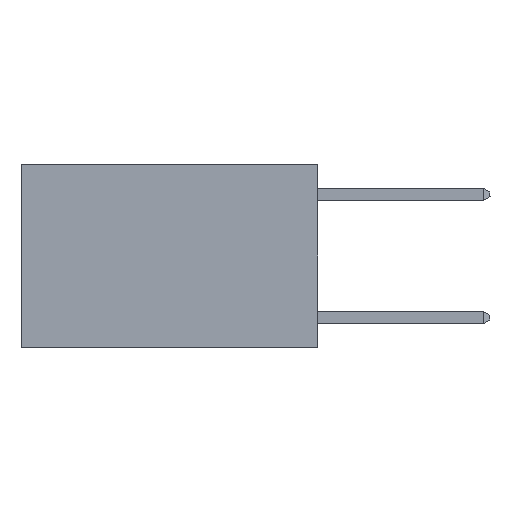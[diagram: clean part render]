
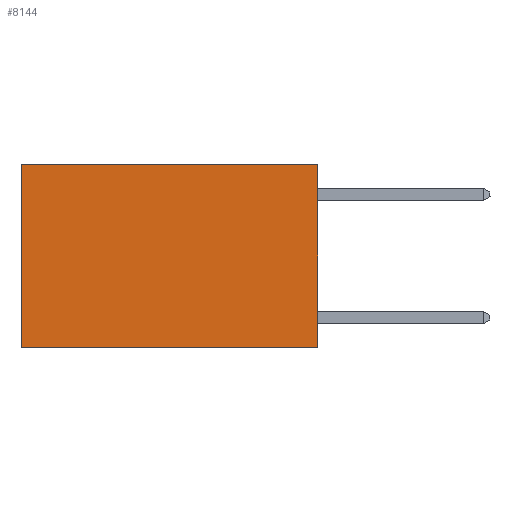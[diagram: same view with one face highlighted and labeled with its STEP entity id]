
A CAD part, left-side view. The second image highlights one B-rep face of the part: STEP entity #8144.
In plain terms, the highlighted planar face has unit normal (-1, 0, 0).
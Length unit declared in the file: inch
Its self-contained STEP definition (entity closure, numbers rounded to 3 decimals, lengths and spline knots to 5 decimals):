
#30 = CARTESIAN_POINT ( 'NONE',  ( 0.2625, 0., -0.37 ) ) ;
#189 = DIRECTION ( 'NONE',  ( 1., 0., 0. ) ) ;
#194 = VERTEX_POINT ( 'NONE', #30 ) ;
#814 = ORIENTED_EDGE ( 'NONE', *, *, #2153, .T. ) ;
#932 = LINE ( 'NONE', #3936, #7458 ) ;
#1233 = DIRECTION ( 'NONE',  ( 0., 0., -1. ) ) ;
#1287 = CARTESIAN_POINT ( 'NONE',  ( 0.2625, 0., 0. ) ) ;
#1314 = LINE ( 'NONE', #4947, #5016 ) ;
#1504 = EDGE_CURVE ( 'NONE', #5482, #5276, #9960, .T. ) ;
#1632 = ORIENTED_EDGE ( 'NONE', *, *, #2874, .F. ) ;
#1901 = VERTEX_POINT ( 'NONE', #2860 ) ;
#2153 = EDGE_CURVE ( 'NONE', #1901, #5482, #1314, .T. ) ;
#2515 = AXIS2_PLACEMENT_3D ( 'NONE', #4694, #189, #10886 ) ;
#2836 = ORIENTED_EDGE ( 'NONE', *, *, #3084, .F. ) ;
#2856 = ORIENTED_EDGE ( 'NONE', *, *, #1504, .T. ) ;
#2860 = CARTESIAN_POINT ( 'NONE',  ( 0.2625, 0., 0. ) ) ;
#2874 = EDGE_CURVE ( 'NONE', #194, #5276, #932, .T. ) ;
#3084 = EDGE_CURVE ( 'NONE', #1901, #194, #3899, .T. ) ;
#3603 = DIRECTION ( 'NONE',  ( 0., 1., 0. ) ) ;
#3899 = LINE ( 'NONE', #1287, #6751 ) ;
#3936 = CARTESIAN_POINT ( 'NONE',  ( 0.2625, 0., -0.37 ) ) ;
#4036 = DIRECTION ( 'NONE',  ( 0., 1., 0. ) ) ;
#4595 = CARTESIAN_POINT ( 'NONE',  ( 0.2625, 0.6, -0.37 ) ) ;
#4597 = VECTOR ( 'NONE', #8091, 39.37008 ) ;
#4694 = CARTESIAN_POINT ( 'NONE',  ( 0.2625, 0., 0. ) ) ;
#4947 = CARTESIAN_POINT ( 'NONE',  ( 0.2625, 0., 0. ) ) ;
#5016 = VECTOR ( 'NONE', #4036, 39.37008 ) ;
#5276 = VERTEX_POINT ( 'NONE', #4595 ) ;
#5482 = VERTEX_POINT ( 'NONE', #8656 ) ;
#5586 = EDGE_LOOP ( 'NONE', ( #2856, #1632, #2836, #814 ) ) ;
#6751 = VECTOR ( 'NONE', #1233, 39.37008 ) ;
#7458 = VECTOR ( 'NONE', #3603, 39.37008 ) ;
#8091 = DIRECTION ( 'NONE',  ( 0., 0., -1. ) ) ;
#8144 = ADVANCED_FACE ( 'NONE', ( #8997 ), #8304, .F. ) ;
#8304 = PLANE ( 'NONE',  #2515 ) ;
#8656 = CARTESIAN_POINT ( 'NONE',  ( 0.2625, 0.6, 0. ) ) ;
#8997 = FACE_OUTER_BOUND ( 'NONE', #5586, .T. ) ;
#9086 = CARTESIAN_POINT ( 'NONE',  ( 0.2625, 0.6, 0. ) ) ;
#9960 = LINE ( 'NONE', #9086, #4597 ) ;
#10886 = DIRECTION ( 'NONE',  ( 0., 0., -1. ) ) ;
